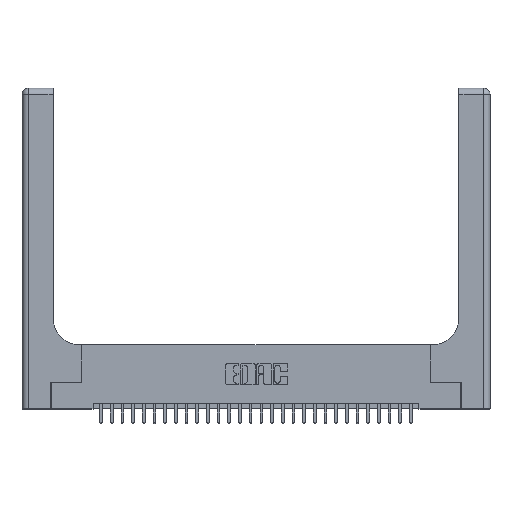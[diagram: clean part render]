
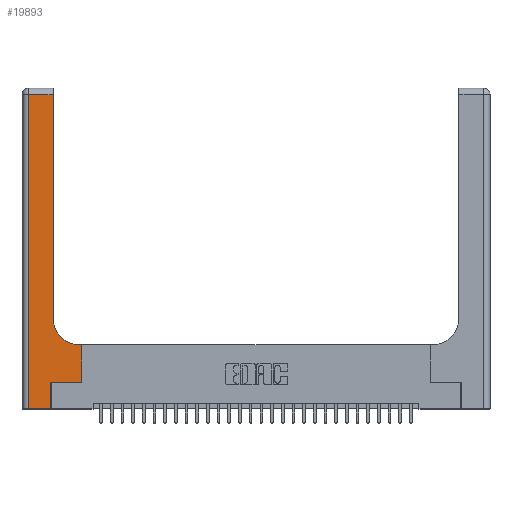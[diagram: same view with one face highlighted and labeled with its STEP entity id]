
A CAD part, top view. The second image highlights one B-rep face of the part: STEP entity #19893.
In plain terms, the highlighted planar face has unit normal (0, 0, 1).
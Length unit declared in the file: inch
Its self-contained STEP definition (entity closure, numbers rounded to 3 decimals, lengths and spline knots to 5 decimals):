
#625 = VERTEX_POINT ( 'NONE', #27307 ) ;
#636 = AXIS2_PLACEMENT_3D ( 'NONE', #23099, #13686, #22796 ) ;
#2242 = CARTESIAN_POINT ( 'NONE',  ( 0.06, 3., 0.37 ) ) ;
#2917 = EDGE_CURVE ( 'NONE', #6688, #25512, #5545, .T. ) ;
#3081 = VERTEX_POINT ( 'NONE', #23850 ) ;
#3180 = CARTESIAN_POINT ( 'NONE',  ( 0., 0., 0.37 ) ) ;
#3202 = CARTESIAN_POINT ( 'NONE',  ( 0., 3., 0.37 ) ) ;
#4044 = EDGE_CURVE ( 'NONE', #11646, #3081, #5101, .T. ) ;
#4377 = VECTOR ( 'NONE', #22402, 39.37008 ) ;
#4651 = VERTEX_POINT ( 'NONE', #21280 ) ;
#4745 = ORIENTED_EDGE ( 'NONE', *, *, #17037, .T. ) ;
#5101 = LINE ( 'NONE', #2242, #29292 ) ;
#5351 = ORIENTED_EDGE ( 'NONE', *, *, #23533, .T. ) ;
#5545 = CIRCLE ( 'NONE', #636, 0.25 ) ;
#6228 = ORIENTED_EDGE ( 'NONE', *, *, #16584, .T. ) ;
#6512 = LINE ( 'NONE', #30112, #28875 ) ;
#6676 = ORIENTED_EDGE ( 'NONE', *, *, #22148, .T. ) ;
#6688 = VERTEX_POINT ( 'NONE', #9748 ) ;
#7280 = LINE ( 'NONE', #10161, #25221 ) ;
#8063 = VECTOR ( 'NONE', #29577, 39.37008 ) ;
#8572 = VECTOR ( 'NONE', #25750, 39.37008 ) ;
#8801 = LINE ( 'NONE', #3180, #4377 ) ;
#8812 = DIRECTION ( 'NONE',  ( -1., 0., 0. ) ) ;
#8986 = EDGE_CURVE ( 'NONE', #3081, #28861, #8801, .T. ) ;
#9186 = CARTESIAN_POINT ( 'NONE',  ( 0.06, 2.94, 0.37 ) ) ;
#9637 = CARTESIAN_POINT ( 'NONE',  ( 0.2915, 0.85, 0.37 ) ) ;
#9748 = CARTESIAN_POINT ( 'NONE',  ( 0.5415, 0.6, 0.37 ) ) ;
#9749 = PLANE ( 'NONE',  #28726 ) ;
#10161 = CARTESIAN_POINT ( 'NONE',  ( 0.2915, 0.6, 0.37 ) ) ;
#10852 = CARTESIAN_POINT ( 'NONE',  ( 0.2915, 3., 0.37 ) ) ;
#11646 = VERTEX_POINT ( 'NONE', #9186 ) ;
#11806 = LINE ( 'NONE', #18960, #8572 ) ;
#12641 = ORIENTED_EDGE ( 'NONE', *, *, #27308, .T. ) ;
#12872 = ORIENTED_EDGE ( 'NONE', *, *, #20909, .T. ) ;
#13116 = ORIENTED_EDGE ( 'NONE', *, *, #4044, .T. ) ;
#13166 = CARTESIAN_POINT ( 'NONE',  ( 0.269, 0.25, 0.37 ) ) ;
#13611 = LINE ( 'NONE', #20771, #18366 ) ;
#13686 = DIRECTION ( 'NONE',  ( 0., 0., -1. ) ) ;
#14679 = CARTESIAN_POINT ( 'NONE',  ( 0.269, 0.25, 0.37 ) ) ;
#15790 = ORIENTED_EDGE ( 'NONE', *, *, #2917, .T. ) ;
#16300 = VECTOR ( 'NONE', #19967, 39.37008 ) ;
#16456 = LINE ( 'NONE', #13166, #8063 ) ;
#16584 = EDGE_CURVE ( 'NONE', #19256, #4651, #16456, .T. ) ;
#17000 = CARTESIAN_POINT ( 'NONE',  ( 0.269, 0., 0.37 ) ) ;
#17037 = EDGE_CURVE ( 'NONE', #30202, #6688, #7280, .T. ) ;
#18366 = VECTOR ( 'NONE', #25708, 39.37008 ) ;
#18960 = CARTESIAN_POINT ( 'NONE',  ( 0.269, 0., 0.37 ) ) ;
#19256 = VERTEX_POINT ( 'NONE', #14679 ) ;
#19893 = ADVANCED_FACE ( 'NONE', ( #29148 ), #9749, .F. ) ;
#19967 = DIRECTION ( 'NONE',  ( 0., 1., 0. ) ) ;
#20771 = CARTESIAN_POINT ( 'NONE',  ( 0.5585, 0.25, 0.37 ) ) ;
#20852 = CARTESIAN_POINT ( 'NONE',  ( 0.5585, 0.6, 0.37 ) ) ;
#20909 = EDGE_CURVE ( 'NONE', #28861, #19256, #11806, .T. ) ;
#21280 = CARTESIAN_POINT ( 'NONE',  ( 0.5585, 0.25, 0.37 ) ) ;
#22112 = DIRECTION ( 'NONE',  ( 0., 0., -1. ) ) ;
#22148 = EDGE_CURVE ( 'NONE', #625, #11646, #6512, .T. ) ;
#22402 = DIRECTION ( 'NONE',  ( 1., 0., 0. ) ) ;
#22796 = DIRECTION ( 'NONE',  ( 1., 0., 0. ) ) ;
#23099 = CARTESIAN_POINT ( 'NONE',  ( 0.5415, 0.85, 0.37 ) ) ;
#23533 = EDGE_CURVE ( 'NONE', #4651, #30202, #13611, .T. ) ;
#23773 = DIRECTION ( 'NONE',  ( -1., 0., 0. ) ) ;
#23850 = CARTESIAN_POINT ( 'NONE',  ( 0.06, 0., 0.37 ) ) ;
#23960 = LINE ( 'NONE', #10852, #16300 ) ;
#24267 = DIRECTION ( 'NONE',  ( -1., 0., 0. ) ) ;
#25221 = VECTOR ( 'NONE', #23773, 39.37008 ) ;
#25512 = VERTEX_POINT ( 'NONE', #9637 ) ;
#25708 = DIRECTION ( 'NONE',  ( 0., 1., 0. ) ) ;
#25750 = DIRECTION ( 'NONE',  ( 0., 1., 0. ) ) ;
#26472 = DIRECTION ( 'NONE',  ( 0., -1., 0. ) ) ;
#27307 = CARTESIAN_POINT ( 'NONE',  ( 0.2915, 2.94, 0.37 ) ) ;
#27308 = EDGE_CURVE ( 'NONE', #25512, #625, #23960, .T. ) ;
#28532 = ORIENTED_EDGE ( 'NONE', *, *, #8986, .T. ) ;
#28726 = AXIS2_PLACEMENT_3D ( 'NONE', #3202, #22112, #24267 ) ;
#28861 = VERTEX_POINT ( 'NONE', #17000 ) ;
#28875 = VECTOR ( 'NONE', #8812, 39.37008 ) ;
#29148 = FACE_OUTER_BOUND ( 'NONE', #29349, .T. ) ;
#29292 = VECTOR ( 'NONE', #26472, 39.37008 ) ;
#29349 = EDGE_LOOP ( 'NONE', ( #12641, #6676, #13116, #28532, #12872, #6228, #5351, #4745, #15790 ) ) ;
#29577 = DIRECTION ( 'NONE',  ( 1., 0., 0. ) ) ;
#30112 = CARTESIAN_POINT ( 'NONE',  ( 0., 2.94, 0.37 ) ) ;
#30202 = VERTEX_POINT ( 'NONE', #20852 ) ;
